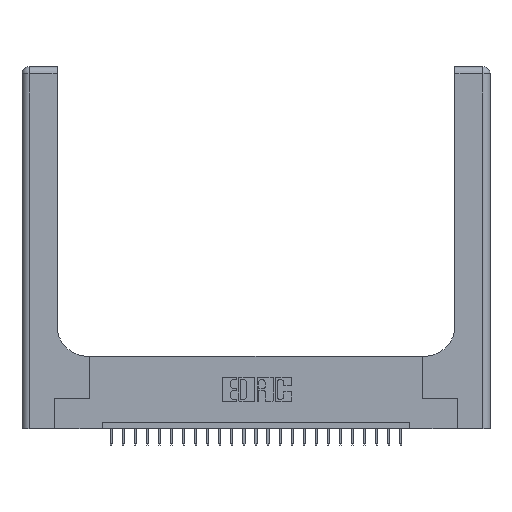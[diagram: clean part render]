
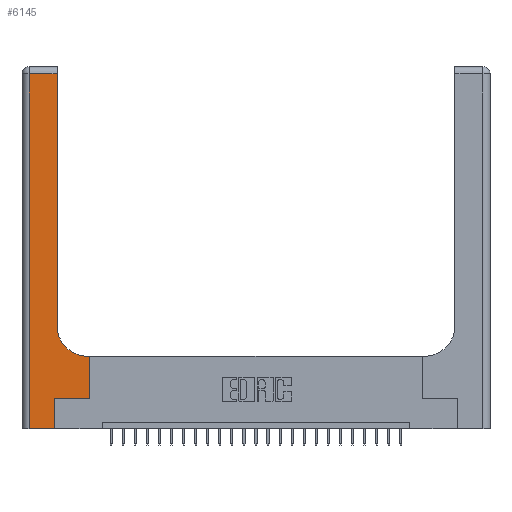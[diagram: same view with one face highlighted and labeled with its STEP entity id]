
A CAD part, top view. The second image highlights one B-rep face of the part: STEP entity #6145.
In plain terms, the highlighted planar face has unit normal (0, 0, 1).
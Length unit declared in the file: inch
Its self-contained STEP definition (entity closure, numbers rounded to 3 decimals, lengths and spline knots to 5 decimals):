
#303 = CARTESIAN_POINT ( 'NONE',  ( 0.5415, 0.6, 0.37 ) ) ;
#782 = VERTEX_POINT ( 'NONE', #303 ) ;
#834 = LINE ( 'NONE', #12591, #21698 ) ;
#1118 = CARTESIAN_POINT ( 'NONE',  ( 0.5585, 0.25, 0.37 ) ) ;
#1364 = DIRECTION ( 'NONE',  ( 0., 0., -1. ) ) ;
#1495 = DIRECTION ( 'NONE',  ( 1., 0., 0. ) ) ;
#1846 = EDGE_CURVE ( 'NONE', #8996, #6237, #12197, .T. ) ;
#1884 = AXIS2_PLACEMENT_3D ( 'NONE', #7636, #23895, #1495 ) ;
#1992 = VERTEX_POINT ( 'NONE', #2582 ) ;
#2252 = CARTESIAN_POINT ( 'NONE',  ( 0.2915, 0.85, 0.37 ) ) ;
#2582 = CARTESIAN_POINT ( 'NONE',  ( 0.06, 0., 0.37 ) ) ;
#2695 = VERTEX_POINT ( 'NONE', #15615 ) ;
#3013 = VECTOR ( 'NONE', #12904, 39.37008 ) ;
#3425 = CARTESIAN_POINT ( 'NONE',  ( 0.269, 0.25, 0.37 ) ) ;
#3971 = DIRECTION ( 'NONE',  ( 1., 0., 0. ) ) ;
#4266 = CARTESIAN_POINT ( 'NONE',  ( 0.5585, 0.25, 0.37 ) ) ;
#4371 = CARTESIAN_POINT ( 'NONE',  ( 0.269, 0.25, 0.37 ) ) ;
#4406 = ORIENTED_EDGE ( 'NONE', *, *, #5816, .T. ) ;
#4436 = CIRCLE ( 'NONE', #1884, 0.25 ) ;
#4704 = ORIENTED_EDGE ( 'NONE', *, *, #9589, .T. ) ;
#4845 = DIRECTION ( 'NONE',  ( 1., 0., 0. ) ) ;
#5064 = EDGE_CURVE ( 'NONE', #10007, #7402, #21055, .T. ) ;
#5365 = CARTESIAN_POINT ( 'NONE',  ( 0., 3., 0.37 ) ) ;
#5569 = CARTESIAN_POINT ( 'NONE',  ( 0.2915, 0.6, 0.37 ) ) ;
#5816 = EDGE_CURVE ( 'NONE', #6237, #17303, #16448, .T. ) ;
#6145 = ADVANCED_FACE ( 'NONE', ( #23633 ), #23361, .F. ) ;
#6237 = VERTEX_POINT ( 'NONE', #24141 ) ;
#7219 = ORIENTED_EDGE ( 'NONE', *, *, #1846, .T. ) ;
#7402 = VERTEX_POINT ( 'NONE', #18418 ) ;
#7636 = CARTESIAN_POINT ( 'NONE',  ( 0.5415, 0.85, 0.37 ) ) ;
#8996 = VERTEX_POINT ( 'NONE', #2252 ) ;
#9589 = EDGE_CURVE ( 'NONE', #2695, #24853, #19145, .T. ) ;
#9680 = VECTOR ( 'NONE', #10804, 39.37008 ) ;
#10007 = VERTEX_POINT ( 'NONE', #1118 ) ;
#10097 = VECTOR ( 'NONE', #15014, 39.37008 ) ;
#10133 = AXIS2_PLACEMENT_3D ( 'NONE', #5365, #1364, #13251 ) ;
#10804 = DIRECTION ( 'NONE',  ( 0., 1., 0. ) ) ;
#11789 = DIRECTION ( 'NONE',  ( 0., 1., 0. ) ) ;
#12197 = LINE ( 'NONE', #24048, #22710 ) ;
#12258 = ORIENTED_EDGE ( 'NONE', *, *, #12401, .T. ) ;
#12401 = EDGE_CURVE ( 'NONE', #24853, #10007, #20218, .T. ) ;
#12529 = ORIENTED_EDGE ( 'NONE', *, *, #5064, .T. ) ;
#12591 = CARTESIAN_POINT ( 'NONE',  ( 0., 0., 0.37 ) ) ;
#12904 = DIRECTION ( 'NONE',  ( 0., 1., 0. ) ) ;
#13251 = DIRECTION ( 'NONE',  ( -1., 0., 0. ) ) ;
#14804 = VECTOR ( 'NONE', #24311, 39.37008 ) ;
#14898 = CARTESIAN_POINT ( 'NONE',  ( 0.269, 0., 0.37 ) ) ;
#14946 = EDGE_LOOP ( 'NONE', ( #7219, #4406, #25369, #20305, #4704, #12258, #12529, #23882, #19852 ) ) ;
#15014 = DIRECTION ( 'NONE',  ( 0., -1., 0. ) ) ;
#15615 = CARTESIAN_POINT ( 'NONE',  ( 0.269, 0., 0.37 ) ) ;
#16448 = LINE ( 'NONE', #26318, #14804 ) ;
#16900 = EDGE_CURVE ( 'NONE', #782, #8996, #4436, .T. ) ;
#16950 = CARTESIAN_POINT ( 'NONE',  ( 0.06, 2.94, 0.37 ) ) ;
#17303 = VERTEX_POINT ( 'NONE', #16950 ) ;
#18418 = CARTESIAN_POINT ( 'NONE',  ( 0.5585, 0.6, 0.37 ) ) ;
#18997 = CARTESIAN_POINT ( 'NONE',  ( 0.06, 3., 0.37 ) ) ;
#19018 = EDGE_CURVE ( 'NONE', #17303, #1992, #25127, .T. ) ;
#19145 = LINE ( 'NONE', #14898, #3013 ) ;
#19158 = VECTOR ( 'NONE', #26094, 39.37008 ) ;
#19852 = ORIENTED_EDGE ( 'NONE', *, *, #16900, .T. ) ;
#20218 = LINE ( 'NONE', #4371, #25648 ) ;
#20305 = ORIENTED_EDGE ( 'NONE', *, *, #24195, .T. ) ;
#21055 = LINE ( 'NONE', #4266, #9680 ) ;
#21698 = VECTOR ( 'NONE', #4845, 39.37008 ) ;
#22710 = VECTOR ( 'NONE', #11789, 39.37008 ) ;
#23361 = PLANE ( 'NONE',  #10133 ) ;
#23633 = FACE_OUTER_BOUND ( 'NONE', #14946, .T. ) ;
#23819 = LINE ( 'NONE', #5569, #19158 ) ;
#23882 = ORIENTED_EDGE ( 'NONE', *, *, #24892, .T. ) ;
#23895 = DIRECTION ( 'NONE',  ( 0., 0., -1. ) ) ;
#24048 = CARTESIAN_POINT ( 'NONE',  ( 0.2915, 3., 0.37 ) ) ;
#24141 = CARTESIAN_POINT ( 'NONE',  ( 0.2915, 2.94, 0.37 ) ) ;
#24195 = EDGE_CURVE ( 'NONE', #1992, #2695, #834, .T. ) ;
#24311 = DIRECTION ( 'NONE',  ( -1., 0., 0. ) ) ;
#24853 = VERTEX_POINT ( 'NONE', #3425 ) ;
#24892 = EDGE_CURVE ( 'NONE', #7402, #782, #23819, .T. ) ;
#25127 = LINE ( 'NONE', #18997, #10097 ) ;
#25369 = ORIENTED_EDGE ( 'NONE', *, *, #19018, .T. ) ;
#25648 = VECTOR ( 'NONE', #3971, 39.37008 ) ;
#26094 = DIRECTION ( 'NONE',  ( -1., 0., 0. ) ) ;
#26318 = CARTESIAN_POINT ( 'NONE',  ( 0., 2.94, 0.37 ) ) ;
